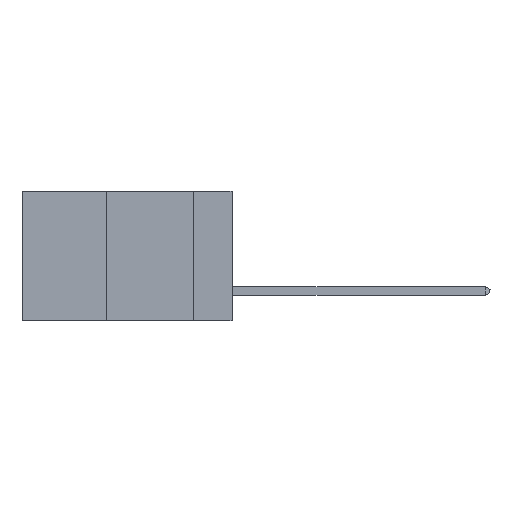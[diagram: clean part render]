
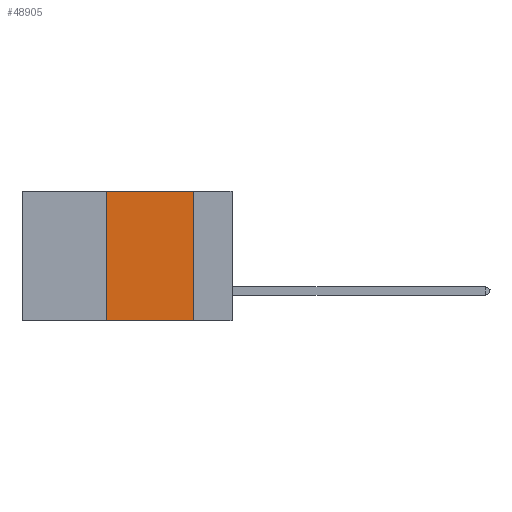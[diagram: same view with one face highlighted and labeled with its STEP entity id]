
A CAD part, left-side view. The second image highlights one B-rep face of the part: STEP entity #48905.
In plain terms, the highlighted planar face has unit normal (-1, 0, 0).
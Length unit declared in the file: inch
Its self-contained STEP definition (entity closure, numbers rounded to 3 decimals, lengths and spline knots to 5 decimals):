
#398 = DIRECTION ( 'NONE',  ( 0., -1., 0. ) ) ;
#633 = DIRECTION ( 'NONE',  ( 0., 0., -1. ) ) ;
#1690 = VERTEX_POINT ( 'NONE', #34317 ) ;
#3945 = CARTESIAN_POINT ( 'NONE',  ( 0., 0.11, -0.37 ) ) ;
#4154 = EDGE_LOOP ( 'NONE', ( #42866, #14489, #7946, #47758 ) ) ;
#4802 = EDGE_CURVE ( 'NONE', #1690, #39631, #9630, .T. ) ;
#7218 = VECTOR ( 'NONE', #398, 39.37008 ) ;
#7946 = ORIENTED_EDGE ( 'NONE', *, *, #25873, .F. ) ;
#9630 = LINE ( 'NONE', #43506, #49095 ) ;
#11961 = DIRECTION ( 'NONE',  ( 0., -1., 0. ) ) ;
#12104 = VERTEX_POINT ( 'NONE', #35540 ) ;
#13451 = LINE ( 'NONE', #44599, #32952 ) ;
#14489 = ORIENTED_EDGE ( 'NONE', *, *, #26687, .F. ) ;
#14938 = EDGE_CURVE ( 'NONE', #12104, #39631, #13451, .T. ) ;
#15627 = AXIS2_PLACEMENT_3D ( 'NONE', #19924, #16499, #633 ) ;
#16172 = PLANE ( 'NONE',  #15627 ) ;
#16499 = DIRECTION ( 'NONE',  ( 1., 0., 0. ) ) ;
#19861 = LINE ( 'NONE', #27361, #7218 ) ;
#19924 = CARTESIAN_POINT ( 'NONE',  ( 0., 0.6, 0. ) ) ;
#25002 = CARTESIAN_POINT ( 'NONE',  ( 0., 0.36, 0. ) ) ;
#25873 = EDGE_CURVE ( 'NONE', #1690, #39556, #31507, .T. ) ;
#26384 = DIRECTION ( 'NONE',  ( 0., 0., 1. ) ) ;
#26687 = EDGE_CURVE ( 'NONE', #39556, #12104, #19861, .T. ) ;
#27361 = CARTESIAN_POINT ( 'NONE',  ( 0., 0.6, 0. ) ) ;
#27795 = FACE_OUTER_BOUND ( 'NONE', #4154, .T. ) ;
#29034 = VECTOR ( 'NONE', #26384, 39.37008 ) ;
#31507 = LINE ( 'NONE', #25002, #29034 ) ;
#32952 = VECTOR ( 'NONE', #41228, 39.37008 ) ;
#34014 = CARTESIAN_POINT ( 'NONE',  ( 0., 0.36, 0. ) ) ;
#34317 = CARTESIAN_POINT ( 'NONE',  ( 0., 0.36, -0.37 ) ) ;
#35540 = CARTESIAN_POINT ( 'NONE',  ( 0., 0.11, 0. ) ) ;
#39556 = VERTEX_POINT ( 'NONE', #34014 ) ;
#39631 = VERTEX_POINT ( 'NONE', #3945 ) ;
#41228 = DIRECTION ( 'NONE',  ( 0., 0., -1. ) ) ;
#42866 = ORIENTED_EDGE ( 'NONE', *, *, #14938, .F. ) ;
#43506 = CARTESIAN_POINT ( 'NONE',  ( 0., 0.6, -0.37 ) ) ;
#44599 = CARTESIAN_POINT ( 'NONE',  ( 0., 0.11, 0. ) ) ;
#47758 = ORIENTED_EDGE ( 'NONE', *, *, #4802, .T. ) ;
#48905 = ADVANCED_FACE ( 'NONE', ( #27795 ), #16172, .F. ) ;
#49095 = VECTOR ( 'NONE', #11961, 39.37008 ) ;
